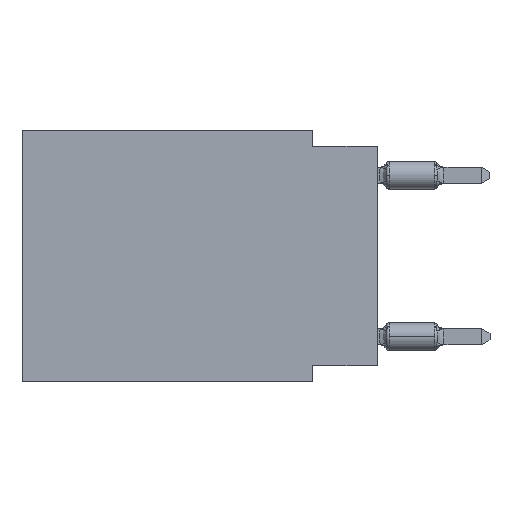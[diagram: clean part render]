
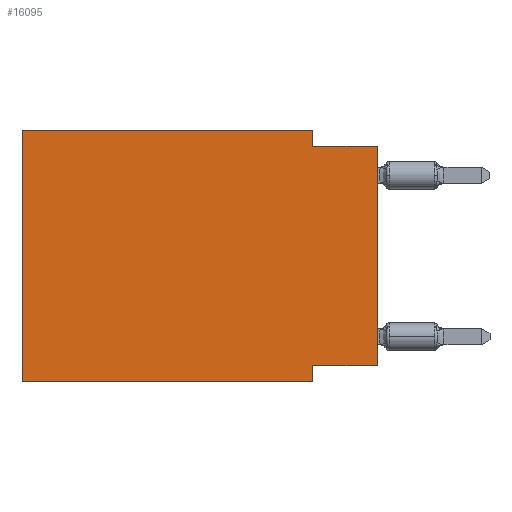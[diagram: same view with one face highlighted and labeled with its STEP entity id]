
A CAD part, left-side view. The second image highlights one B-rep face of the part: STEP entity #16095.
In plain terms, the highlighted planar face has unit normal (-1, 0, 0).
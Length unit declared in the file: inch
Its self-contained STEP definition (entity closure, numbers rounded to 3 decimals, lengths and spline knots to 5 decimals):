
#910 = CARTESIAN_POINT ( 'NONE',  ( 0., 0.1, -0.39 ) ) ;
#1004 = CARTESIAN_POINT ( 'NONE',  ( 0., 0.55, 0. ) ) ;
#1161 = VECTOR ( 'NONE', #5662, 39.37008 ) ;
#1331 = DIRECTION ( 'NONE',  ( 0., -1., 0. ) ) ;
#1780 = VERTEX_POINT ( 'NONE', #16211 ) ;
#2028 = DIRECTION ( 'NONE',  ( 0., 1., 0. ) ) ;
#2184 = DIRECTION ( 'NONE',  ( 1., 0., 0. ) ) ;
#2731 = VECTOR ( 'NONE', #1331, 39.37008 ) ;
#3253 = CARTESIAN_POINT ( 'NONE',  ( 0., 0., -0.025 ) ) ;
#3610 = CARTESIAN_POINT ( 'NONE',  ( 0., 0.1, 0. ) ) ;
#4068 = ORIENTED_EDGE ( 'NONE', *, *, #14036, .F. ) ;
#4162 = LINE ( 'NONE', #17316, #2731 ) ;
#4206 = EDGE_CURVE ( 'NONE', #6012, #8881, #16491, .T. ) ;
#4228 = CARTESIAN_POINT ( 'NONE',  ( 0., 0.1, 0. ) ) ;
#4941 = CARTESIAN_POINT ( 'NONE',  ( 0., 0.55, 0. ) ) ;
#5113 = ORIENTED_EDGE ( 'NONE', *, *, #4206, .F. ) ;
#5141 = CARTESIAN_POINT ( 'NONE',  ( 0., 0., -0.365 ) ) ;
#5157 = VERTEX_POINT ( 'NONE', #1004 ) ;
#5237 = VECTOR ( 'NONE', #11816, 39.37008 ) ;
#5662 = DIRECTION ( 'NONE',  ( 0., 0., 1. ) ) ;
#5861 = CARTESIAN_POINT ( 'NONE',  ( 0., 0.1, -0.025 ) ) ;
#6012 = VERTEX_POINT ( 'NONE', #4228 ) ;
#6350 = LINE ( 'NONE', #4941, #12676 ) ;
#6365 = LINE ( 'NONE', #5141, #17723 ) ;
#6368 = EDGE_CURVE ( 'NONE', #13946, #10084, #13727, .T. ) ;
#6518 = CARTESIAN_POINT ( 'NONE',  ( 0., 0.1, -0.39 ) ) ;
#6643 = DIRECTION ( 'NONE',  ( 0., -1., 0. ) ) ;
#6913 = CARTESIAN_POINT ( 'NONE',  ( 0., 0.55, -0.39 ) ) ;
#6973 = CARTESIAN_POINT ( 'NONE',  ( 0., 0.1, -0.365 ) ) ;
#7049 = VERTEX_POINT ( 'NONE', #13323 ) ;
#7076 = ORIENTED_EDGE ( 'NONE', *, *, #12413, .F. ) ;
#7150 = LINE ( 'NONE', #8849, #10242 ) ;
#7276 = CARTESIAN_POINT ( 'NONE',  ( 0., 0., 0. ) ) ;
#7520 = AXIS2_PLACEMENT_3D ( 'NONE', #15079, #2184, #7942 ) ;
#7633 = ORIENTED_EDGE ( 'NONE', *, *, #11686, .F. ) ;
#7684 = EDGE_CURVE ( 'NONE', #7049, #8143, #10298, .T. ) ;
#7905 = DIRECTION ( 'NONE',  ( 0., 0., -1. ) ) ;
#7942 = DIRECTION ( 'NONE',  ( 0., 0., -1. ) ) ;
#8143 = VERTEX_POINT ( 'NONE', #3253 ) ;
#8756 = VECTOR ( 'NONE', #6643, 39.37008 ) ;
#8849 = CARTESIAN_POINT ( 'NONE',  ( 0., 0.55, 0. ) ) ;
#8881 = VERTEX_POINT ( 'NONE', #5861 ) ;
#9346 = PLANE ( 'NONE',  #7520 ) ;
#9938 = LINE ( 'NONE', #6913, #8756 ) ;
#10084 = VERTEX_POINT ( 'NONE', #6518 ) ;
#10103 = EDGE_LOOP ( 'NONE', ( #16929, #7076, #5113, #17216, #4068, #10224, #15116, #7633 ) ) ;
#10224 = ORIENTED_EDGE ( 'NONE', *, *, #11929, .T. ) ;
#10242 = VECTOR ( 'NONE', #14385, 39.37008 ) ;
#10298 = LINE ( 'NONE', #7276, #1161 ) ;
#11686 = EDGE_CURVE ( 'NONE', #7049, #13946, #6365, .T. ) ;
#11816 = DIRECTION ( 'NONE',  ( 0., 0., -1. ) ) ;
#11929 = EDGE_CURVE ( 'NONE', #1780, #10084, #9938, .T. ) ;
#12413 = EDGE_CURVE ( 'NONE', #8881, #8143, #4162, .T. ) ;
#12676 = VECTOR ( 'NONE', #13780, 39.37008 ) ;
#13323 = CARTESIAN_POINT ( 'NONE',  ( 0., 0., -0.365 ) ) ;
#13727 = LINE ( 'NONE', #910, #17882 ) ;
#13780 = DIRECTION ( 'NONE',  ( 0., -1., 0. ) ) ;
#13946 = VERTEX_POINT ( 'NONE', #6973 ) ;
#14036 = EDGE_CURVE ( 'NONE', #1780, #5157, #7150, .T. ) ;
#14385 = DIRECTION ( 'NONE',  ( 0., 0., 1. ) ) ;
#15079 = CARTESIAN_POINT ( 'NONE',  ( 0., 0.55, 0. ) ) ;
#15116 = ORIENTED_EDGE ( 'NONE', *, *, #6368, .F. ) ;
#15675 = EDGE_CURVE ( 'NONE', #5157, #6012, #6350, .T. ) ;
#16095 = ADVANCED_FACE ( 'NONE', ( #17877 ), #9346, .F. ) ;
#16211 = CARTESIAN_POINT ( 'NONE',  ( 0., 0.55, -0.39 ) ) ;
#16491 = LINE ( 'NONE', #3610, #5237 ) ;
#16929 = ORIENTED_EDGE ( 'NONE', *, *, #7684, .T. ) ;
#17216 = ORIENTED_EDGE ( 'NONE', *, *, #15675, .F. ) ;
#17316 = CARTESIAN_POINT ( 'NONE',  ( 0., 0., -0.025 ) ) ;
#17723 = VECTOR ( 'NONE', #2028, 39.37008 ) ;
#17877 = FACE_OUTER_BOUND ( 'NONE', #10103, .T. ) ;
#17882 = VECTOR ( 'NONE', #7905, 39.37008 ) ;
